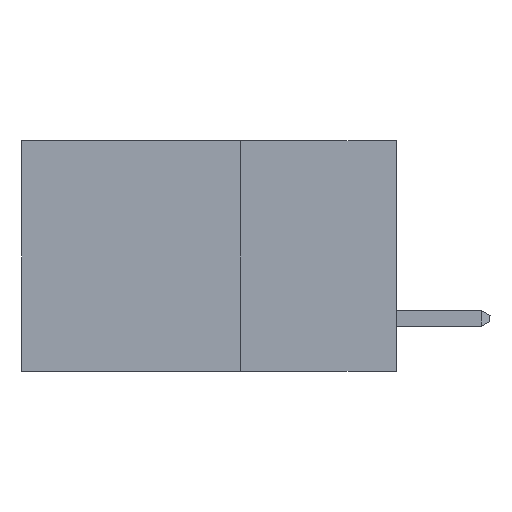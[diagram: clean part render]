
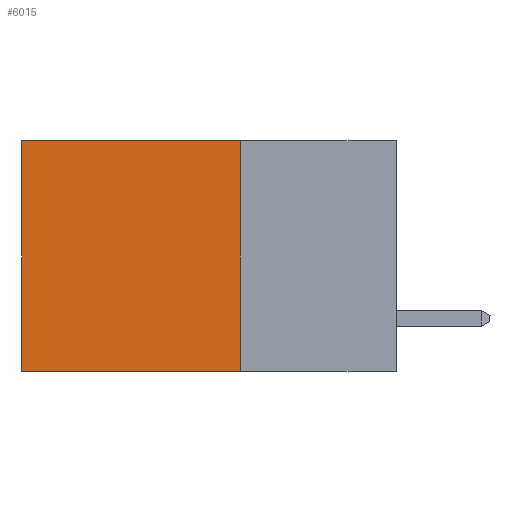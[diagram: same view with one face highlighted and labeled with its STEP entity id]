
A CAD part, left-side view. The second image highlights one B-rep face of the part: STEP entity #6015.
In plain terms, the highlighted planar face has unit normal (-1, 0, 0).
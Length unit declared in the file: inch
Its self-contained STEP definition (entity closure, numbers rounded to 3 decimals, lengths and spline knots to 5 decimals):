
#423 = EDGE_CURVE ( 'NONE', #20548, #12272, #484, .T. ) ;
#480 = EDGE_CURVE ( 'NONE', #13783, #12272, #21571, .T. ) ;
#484 = LINE ( 'NONE', #24980, #20223 ) ;
#636 = EDGE_CURVE ( 'NONE', #20299, #13783, #14259, .T. ) ;
#892 = CARTESIAN_POINT ( 'NONE',  ( 0.2615, 0.25, -0.37 ) ) ;
#3268 = DIRECTION ( 'NONE',  ( 0., 0., -1. ) ) ;
#4035 = CARTESIAN_POINT ( 'NONE',  ( 0.2615, 0.25, 0. ) ) ;
#4184 = ORIENTED_EDGE ( 'NONE', *, *, #480, .T. ) ;
#4318 = ORIENTED_EDGE ( 'NONE', *, *, #11425, .F. ) ;
#4432 = CARTESIAN_POINT ( 'NONE',  ( 0.2615, 0.25, -0.37 ) ) ;
#6015 = ADVANCED_FACE ( 'NONE', ( #9394 ), #19605, .F. ) ;
#6349 = CARTESIAN_POINT ( 'NONE',  ( 0.2615, 0.6, -0.37 ) ) ;
#8338 = VECTOR ( 'NONE', #3268, 39.37008 ) ;
#8363 = ORIENTED_EDGE ( 'NONE', *, *, #423, .F. ) ;
#8534 = LINE ( 'NONE', #4432, #12423 ) ;
#8955 = DIRECTION ( 'NONE',  ( 0., 1., 0. ) ) ;
#9123 = DIRECTION ( 'NONE',  ( 1., 0., 0. ) ) ;
#9394 = FACE_OUTER_BOUND ( 'NONE', #24867, .T. ) ;
#9671 = CARTESIAN_POINT ( 'NONE',  ( 0.2615, 0.25, -0.37 ) ) ;
#10480 = CARTESIAN_POINT ( 'NONE',  ( 0.2615, 0.6, 0. ) ) ;
#10485 = AXIS2_PLACEMENT_3D ( 'NONE', #9671, #9123, #17481 ) ;
#11425 = EDGE_CURVE ( 'NONE', #20299, #20548, #8534, .T. ) ;
#12272 = VERTEX_POINT ( 'NONE', #6349 ) ;
#12423 = VECTOR ( 'NONE', #18103, 39.37008 ) ;
#13783 = VERTEX_POINT ( 'NONE', #10480 ) ;
#14041 = CARTESIAN_POINT ( 'NONE',  ( 0.2615, 0.25, 0. ) ) ;
#14259 = LINE ( 'NONE', #4035, #19387 ) ;
#17481 = DIRECTION ( 'NONE',  ( 0., 0., -1. ) ) ;
#18103 = DIRECTION ( 'NONE',  ( 0., 0., -1. ) ) ;
#19387 = VECTOR ( 'NONE', #24424, 39.37008 ) ;
#19605 = PLANE ( 'NONE',  #10485 ) ;
#19838 = CARTESIAN_POINT ( 'NONE',  ( 0.2615, 0.6, -0.37 ) ) ;
#20223 = VECTOR ( 'NONE', #8955, 39.37008 ) ;
#20299 = VERTEX_POINT ( 'NONE', #14041 ) ;
#20548 = VERTEX_POINT ( 'NONE', #892 ) ;
#20795 = ORIENTED_EDGE ( 'NONE', *, *, #636, .T. ) ;
#21571 = LINE ( 'NONE', #19838, #8338 ) ;
#24424 = DIRECTION ( 'NONE',  ( 0., 1., 0. ) ) ;
#24867 = EDGE_LOOP ( 'NONE', ( #4184, #8363, #4318, #20795 ) ) ;
#24980 = CARTESIAN_POINT ( 'NONE',  ( 0.2615, 0.25, -0.37 ) ) ;
